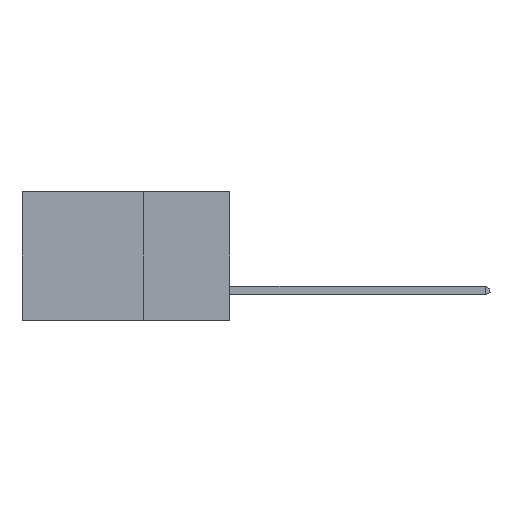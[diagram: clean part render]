
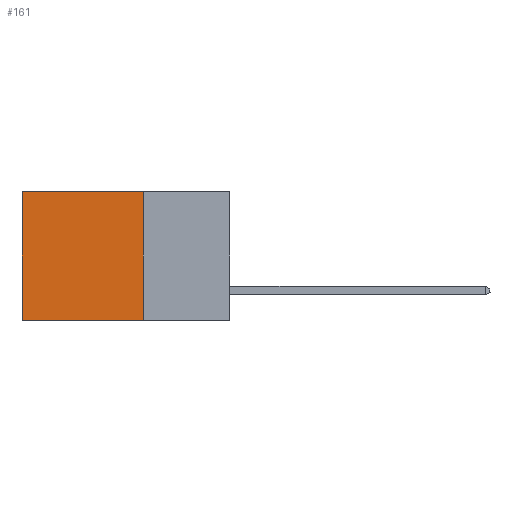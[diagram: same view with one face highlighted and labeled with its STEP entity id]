
A CAD part, left-side view. The second image highlights one B-rep face of the part: STEP entity #161.
In plain terms, the highlighted planar face has unit normal (-1, 0, 0).
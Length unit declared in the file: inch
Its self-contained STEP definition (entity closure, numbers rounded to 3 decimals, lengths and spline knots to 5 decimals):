
#161 = ADVANCED_FACE ( 'NONE', ( #2825 ), #11436, .F. ) ;
#526 = ORIENTED_EDGE ( 'NONE', *, *, #22576, .T. ) ;
#1166 = DIRECTION ( 'NONE',  ( 0., 0., -1. ) ) ;
#2326 = ORIENTED_EDGE ( 'NONE', *, *, #28481, .F. ) ;
#2825 = FACE_OUTER_BOUND ( 'NONE', #3347, .T. ) ;
#3347 = EDGE_LOOP ( 'NONE', ( #6304, #2326, #17018, #526 ) ) ;
#3974 = VECTOR ( 'NONE', #14699, 39.37008 ) ;
#5653 = VECTOR ( 'NONE', #28438, 39.37008 ) ;
#6059 = LINE ( 'NONE', #27842, #8827 ) ;
#6304 = ORIENTED_EDGE ( 'NONE', *, *, #19894, .T. ) ;
#6999 = LINE ( 'NONE', #8458, #18962 ) ;
#8061 = CARTESIAN_POINT ( 'NONE',  ( 0.298, 0.25, -0.37 ) ) ;
#8458 = CARTESIAN_POINT ( 'NONE',  ( 0.298, 0.25, 0. ) ) ;
#8827 = VECTOR ( 'NONE', #1166, 39.37008 ) ;
#11308 = CARTESIAN_POINT ( 'NONE',  ( 0.298, 0.6, 0. ) ) ;
#11436 = PLANE ( 'NONE',  #19209 ) ;
#11873 = VERTEX_POINT ( 'NONE', #28475 ) ;
#11884 = LINE ( 'NONE', #18995, #3974 ) ;
#13661 = DIRECTION ( 'NONE',  ( 0., 0., -1. ) ) ;
#14289 = LINE ( 'NONE', #8061, #5653 ) ;
#14699 = DIRECTION ( 'NONE',  ( 0., 0., -1. ) ) ;
#16233 = VERTEX_POINT ( 'NONE', #11308 ) ;
#17018 = ORIENTED_EDGE ( 'NONE', *, *, #20508, .F. ) ;
#17511 = CARTESIAN_POINT ( 'NONE',  ( 0.298, 0.6, -0.37 ) ) ;
#18962 = VECTOR ( 'NONE', #28272, 39.37008 ) ;
#18995 = CARTESIAN_POINT ( 'NONE',  ( 0.298, 0.25, 0. ) ) ;
#19209 = AXIS2_PLACEMENT_3D ( 'NONE', #24602, #26729, #13661 ) ;
#19894 = EDGE_CURVE ( 'NONE', #16233, #28202, #6059, .T. ) ;
#20508 = EDGE_CURVE ( 'NONE', #22592, #11873, #11884, .T. ) ;
#22576 = EDGE_CURVE ( 'NONE', #22592, #16233, #6999, .T. ) ;
#22592 = VERTEX_POINT ( 'NONE', #26036 ) ;
#24602 = CARTESIAN_POINT ( 'NONE',  ( 0.298, 0.25, 0. ) ) ;
#26036 = CARTESIAN_POINT ( 'NONE',  ( 0.298, 0.25, 0. ) ) ;
#26729 = DIRECTION ( 'NONE',  ( 1., 0., 0. ) ) ;
#27842 = CARTESIAN_POINT ( 'NONE',  ( 0.298, 0.6, 0. ) ) ;
#28202 = VERTEX_POINT ( 'NONE', #17511 ) ;
#28272 = DIRECTION ( 'NONE',  ( 0., 1., 0. ) ) ;
#28438 = DIRECTION ( 'NONE',  ( 0., 1., 0. ) ) ;
#28475 = CARTESIAN_POINT ( 'NONE',  ( 0.298, 0.25, -0.37 ) ) ;
#28481 = EDGE_CURVE ( 'NONE', #11873, #28202, #14289, .T. ) ;
